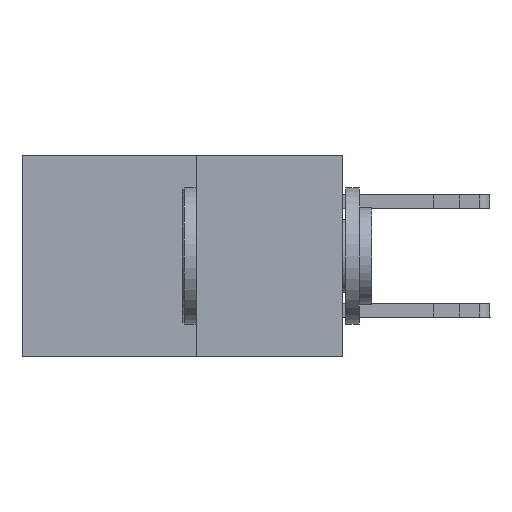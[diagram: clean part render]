
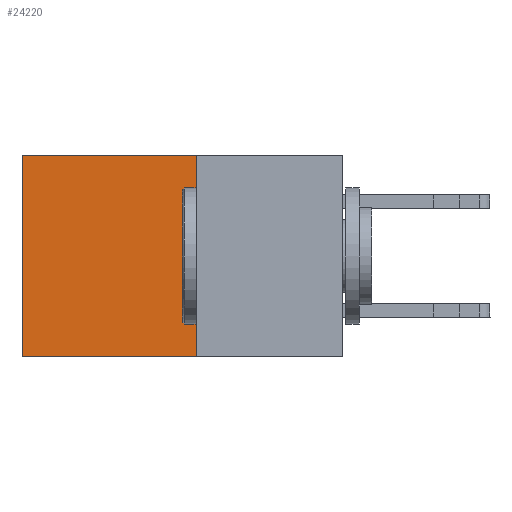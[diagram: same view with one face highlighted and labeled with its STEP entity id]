
A CAD part, left-side view. The second image highlights one B-rep face of the part: STEP entity #24220.
In plain terms, the highlighted planar face has unit normal (-1, 0, 0).
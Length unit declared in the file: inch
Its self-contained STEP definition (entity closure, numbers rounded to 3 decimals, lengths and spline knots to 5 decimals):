
#263 = PLANE ( 'NONE',  #9850 ) ;
#1638 = DIRECTION ( 'NONE',  ( 0., 1., 0. ) ) ;
#1739 = EDGE_CURVE ( 'NONE', #23824, #22580, #23783, .T. ) ;
#1920 = CARTESIAN_POINT ( 'NONE',  ( 0.277, 0.59, 0. ) ) ;
#2502 = CARTESIAN_POINT ( 'NONE',  ( 0.277, 0.59, -0.37 ) ) ;
#3588 = VERTEX_POINT ( 'NONE', #27664 ) ;
#5098 = DIRECTION ( 'NONE',  ( 0., 0., -1. ) ) ;
#5599 = CARTESIAN_POINT ( 'NONE',  ( 0.277, 0.27, -0.37 ) ) ;
#6136 = CARTESIAN_POINT ( 'NONE',  ( 0.277, 0.27, -0.37 ) ) ;
#8556 = DIRECTION ( 'NONE',  ( 0., 1., 0. ) ) ;
#9782 = DIRECTION ( 'NONE',  ( 0., 0., -1. ) ) ;
#9850 = AXIS2_PLACEMENT_3D ( 'NONE', #17090, #19527, #5098 ) ;
#10700 = VECTOR ( 'NONE', #20038, 39.37008 ) ;
#10763 = ORIENTED_EDGE ( 'NONE', *, *, #23461, .T. ) ;
#10986 = VERTEX_POINT ( 'NONE', #16033 ) ;
#11020 = VECTOR ( 'NONE', #1638, 39.37008 ) ;
#11778 = VECTOR ( 'NONE', #9782, 39.37008 ) ;
#12003 = ORIENTED_EDGE ( 'NONE', *, *, #1739, .T. ) ;
#12525 = CARTESIAN_POINT ( 'NONE',  ( 0.277, 0.27, 0. ) ) ;
#14581 = EDGE_LOOP ( 'NONE', ( #10763, #19300, #18471, #12003 ) ) ;
#15488 = FACE_OUTER_BOUND ( 'NONE', #14581, .T. ) ;
#16033 = CARTESIAN_POINT ( 'NONE',  ( 0.277, 0.59, -0.37 ) ) ;
#16260 = EDGE_CURVE ( 'NONE', #3588, #10986, #19356, .T. ) ;
#17090 = CARTESIAN_POINT ( 'NONE',  ( 0.277, 0.27, -0.37 ) ) ;
#17434 = LINE ( 'NONE', #2502, #11778 ) ;
#18471 = ORIENTED_EDGE ( 'NONE', *, *, #30006, .F. ) ;
#19300 = ORIENTED_EDGE ( 'NONE', *, *, #16260, .F. ) ;
#19356 = LINE ( 'NONE', #6136, #23436 ) ;
#19527 = DIRECTION ( 'NONE',  ( 1., 0., 0. ) ) ;
#20038 = DIRECTION ( 'NONE',  ( 0., 0., -1. ) ) ;
#22580 = VERTEX_POINT ( 'NONE', #1920 ) ;
#22870 = CARTESIAN_POINT ( 'NONE',  ( 0.277, 0.27, 0. ) ) ;
#23436 = VECTOR ( 'NONE', #8556, 39.37008 ) ;
#23445 = LINE ( 'NONE', #5599, #10700 ) ;
#23461 = EDGE_CURVE ( 'NONE', #22580, #10986, #17434, .T. ) ;
#23783 = LINE ( 'NONE', #12525, #11020 ) ;
#23824 = VERTEX_POINT ( 'NONE', #22870 ) ;
#24220 = ADVANCED_FACE ( 'NONE', ( #15488 ), #263, .F. ) ;
#27664 = CARTESIAN_POINT ( 'NONE',  ( 0.277, 0.27, -0.37 ) ) ;
#30006 = EDGE_CURVE ( 'NONE', #23824, #3588, #23445, .T. ) ;
